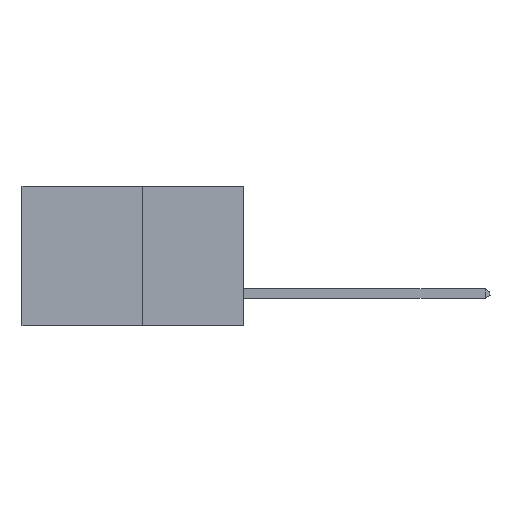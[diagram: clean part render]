
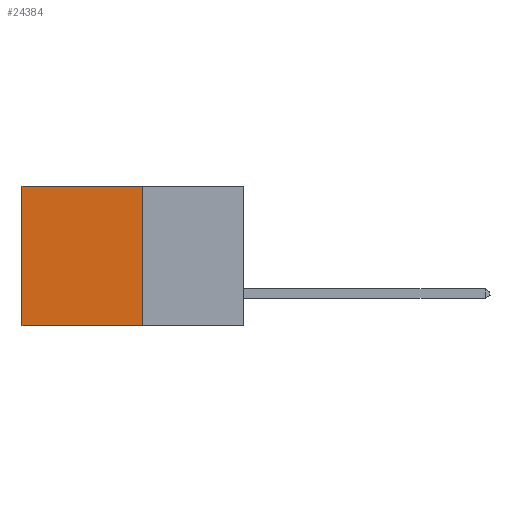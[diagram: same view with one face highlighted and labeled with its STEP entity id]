
A CAD part, left-side view. The second image highlights one B-rep face of the part: STEP entity #24384.
In plain terms, the highlighted planar face has unit normal (-1, 0, 0).
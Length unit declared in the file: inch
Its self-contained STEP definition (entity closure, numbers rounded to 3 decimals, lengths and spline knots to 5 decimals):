
#537 = CARTESIAN_POINT ( 'NONE',  ( 0.277, 0.27, -0.37 ) ) ;
#907 = CARTESIAN_POINT ( 'NONE',  ( 0.277, 0.27, -0.37 ) ) ;
#962 = AXIS2_PLACEMENT_3D ( 'NONE', #8665, #19771, #6542 ) ;
#1712 = FACE_OUTER_BOUND ( 'NONE', #12651, .T. ) ;
#3155 = DIRECTION ( 'NONE',  ( 0., 1., 0. ) ) ;
#3319 = ORIENTED_EDGE ( 'NONE', *, *, #3744, .T. ) ;
#3744 = EDGE_CURVE ( 'NONE', #21757, #6924, #23805, .T. ) ;
#4232 = VECTOR ( 'NONE', #11603, 39.37008 ) ;
#4325 = PLANE ( 'NONE',  #962 ) ;
#6542 = DIRECTION ( 'NONE',  ( 0., 0., -1. ) ) ;
#6924 = VERTEX_POINT ( 'NONE', #19414 ) ;
#7550 = VERTEX_POINT ( 'NONE', #11150 ) ;
#7560 = ORIENTED_EDGE ( 'NONE', *, *, #8736, .T. ) ;
#7929 = CARTESIAN_POINT ( 'NONE',  ( 0.277, 0.27, -0.37 ) ) ;
#8665 = CARTESIAN_POINT ( 'NONE',  ( 0.277, 0.27, -0.37 ) ) ;
#8678 = DIRECTION ( 'NONE',  ( 0., 0., -1. ) ) ;
#8736 = EDGE_CURVE ( 'NONE', #7550, #21757, #11871, .T. ) ;
#9695 = CARTESIAN_POINT ( 'NONE',  ( 0.277, 0.59, -0.37 ) ) ;
#10110 = DIRECTION ( 'NONE',  ( 0., 1., 0. ) ) ;
#11150 = CARTESIAN_POINT ( 'NONE',  ( 0.277, 0.27, 0. ) ) ;
#11603 = DIRECTION ( 'NONE',  ( 0., 0., -1. ) ) ;
#11871 = LINE ( 'NONE', #25390, #27899 ) ;
#12212 = VECTOR ( 'NONE', #8678, 39.37008 ) ;
#12651 = EDGE_LOOP ( 'NONE', ( #3319, #17146, #27824, #7560 ) ) ;
#14894 = VECTOR ( 'NONE', #3155, 39.37008 ) ;
#15089 = EDGE_CURVE ( 'NONE', #7550, #27754, #27564, .T. ) ;
#17146 = ORIENTED_EDGE ( 'NONE', *, *, #24726, .F. ) ;
#19414 = CARTESIAN_POINT ( 'NONE',  ( 0.277, 0.59, -0.37 ) ) ;
#19771 = DIRECTION ( 'NONE',  ( 1., 0., 0. ) ) ;
#20697 = LINE ( 'NONE', #907, #14894 ) ;
#21757 = VERTEX_POINT ( 'NONE', #22847 ) ;
#22847 = CARTESIAN_POINT ( 'NONE',  ( 0.277, 0.59, 0. ) ) ;
#23805 = LINE ( 'NONE', #9695, #12212 ) ;
#24384 = ADVANCED_FACE ( 'NONE', ( #1712 ), #4325, .F. ) ;
#24726 = EDGE_CURVE ( 'NONE', #27754, #6924, #20697, .T. ) ;
#25390 = CARTESIAN_POINT ( 'NONE',  ( 0.277, 0.27, 0. ) ) ;
#27564 = LINE ( 'NONE', #537, #4232 ) ;
#27754 = VERTEX_POINT ( 'NONE', #7929 ) ;
#27824 = ORIENTED_EDGE ( 'NONE', *, *, #15089, .F. ) ;
#27899 = VECTOR ( 'NONE', #10110, 39.37008 ) ;
